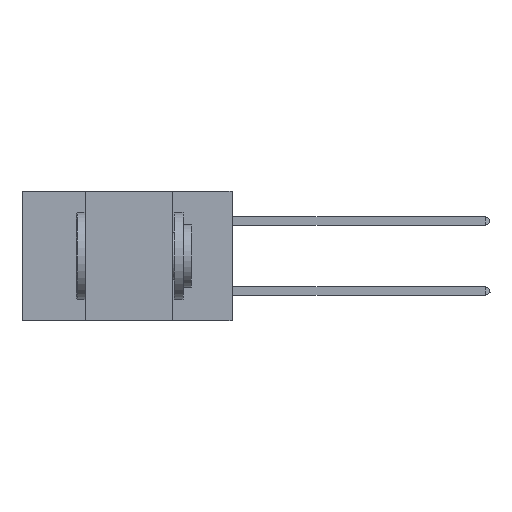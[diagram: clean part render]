
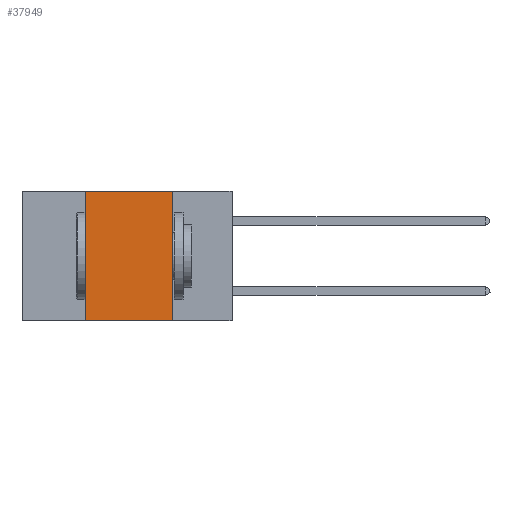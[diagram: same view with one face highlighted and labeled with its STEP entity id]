
A CAD part, left-side view. The second image highlights one B-rep face of the part: STEP entity #37949.
In plain terms, the highlighted planar face has unit normal (-1, 0, 0).
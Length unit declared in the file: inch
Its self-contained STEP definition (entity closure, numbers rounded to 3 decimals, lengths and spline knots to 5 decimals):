
#2822 = EDGE_CURVE ( 'NONE', #17573, #23221, #29398, .T. ) ;
#6019 = EDGE_CURVE ( 'NONE', #39747, #17573, #19993, .T. ) ;
#6937 = DIRECTION ( 'NONE',  ( 1., 0., 0. ) ) ;
#8474 = EDGE_CURVE ( 'NONE', #10605, #23221, #18812, .T. ) ;
#9616 = CARTESIAN_POINT ( 'NONE',  ( 0., 0.42, -0.37 ) ) ;
#10231 = DIRECTION ( 'NONE',  ( 0., 0., 1. ) ) ;
#10500 = CARTESIAN_POINT ( 'NONE',  ( 0., 0.17, 0. ) ) ;
#10605 = VERTEX_POINT ( 'NONE', #9616 ) ;
#13614 = VECTOR ( 'NONE', #10231, 39.37008 ) ;
#14793 = ORIENTED_EDGE ( 'NONE', *, *, #2822, .F. ) ;
#15171 = VECTOR ( 'NONE', #28872, 39.37008 ) ;
#15634 = CARTESIAN_POINT ( 'NONE',  ( 0., 0.17, 0. ) ) ;
#16379 = CARTESIAN_POINT ( 'NONE',  ( 0., 0.6, 0. ) ) ;
#17573 = VERTEX_POINT ( 'NONE', #10500 ) ;
#18812 = LINE ( 'NONE', #19701, #36603 ) ;
#18937 = FACE_OUTER_BOUND ( 'NONE', #24580, .T. ) ;
#19701 = CARTESIAN_POINT ( 'NONE',  ( 0., 0.6, -0.37 ) ) ;
#19775 = DIRECTION ( 'NONE',  ( 0., -1., 0. ) ) ;
#19993 = LINE ( 'NONE', #39566, #36857 ) ;
#20606 = ORIENTED_EDGE ( 'NONE', *, *, #6019, .F. ) ;
#23221 = VERTEX_POINT ( 'NONE', #35984 ) ;
#23333 = LINE ( 'NONE', #33624, #13614 ) ;
#24580 = EDGE_LOOP ( 'NONE', ( #14793, #20606, #37550, #25397 ) ) ;
#25397 = ORIENTED_EDGE ( 'NONE', *, *, #8474, .T. ) ;
#25520 = EDGE_CURVE ( 'NONE', #10605, #39747, #23333, .T. ) ;
#28542 = DIRECTION ( 'NONE',  ( 0., -1., 0. ) ) ;
#28763 = AXIS2_PLACEMENT_3D ( 'NONE', #16379, #6937, #39428 ) ;
#28872 = DIRECTION ( 'NONE',  ( 0., 0., -1. ) ) ;
#29398 = LINE ( 'NONE', #15634, #15171 ) ;
#33624 = CARTESIAN_POINT ( 'NONE',  ( 0., 0.42, 0. ) ) ;
#35984 = CARTESIAN_POINT ( 'NONE',  ( 0., 0.17, -0.37 ) ) ;
#36434 = PLANE ( 'NONE',  #28763 ) ;
#36603 = VECTOR ( 'NONE', #28542, 39.37008 ) ;
#36857 = VECTOR ( 'NONE', #19775, 39.37008 ) ;
#37550 = ORIENTED_EDGE ( 'NONE', *, *, #25520, .F. ) ;
#37949 = ADVANCED_FACE ( 'NONE', ( #18937 ), #36434, .F. ) ;
#39428 = DIRECTION ( 'NONE',  ( 0., 0., -1. ) ) ;
#39566 = CARTESIAN_POINT ( 'NONE',  ( 0., 0.6, 0. ) ) ;
#39747 = VERTEX_POINT ( 'NONE', #39909 ) ;
#39909 = CARTESIAN_POINT ( 'NONE',  ( 0., 0.42, 0. ) ) ;
